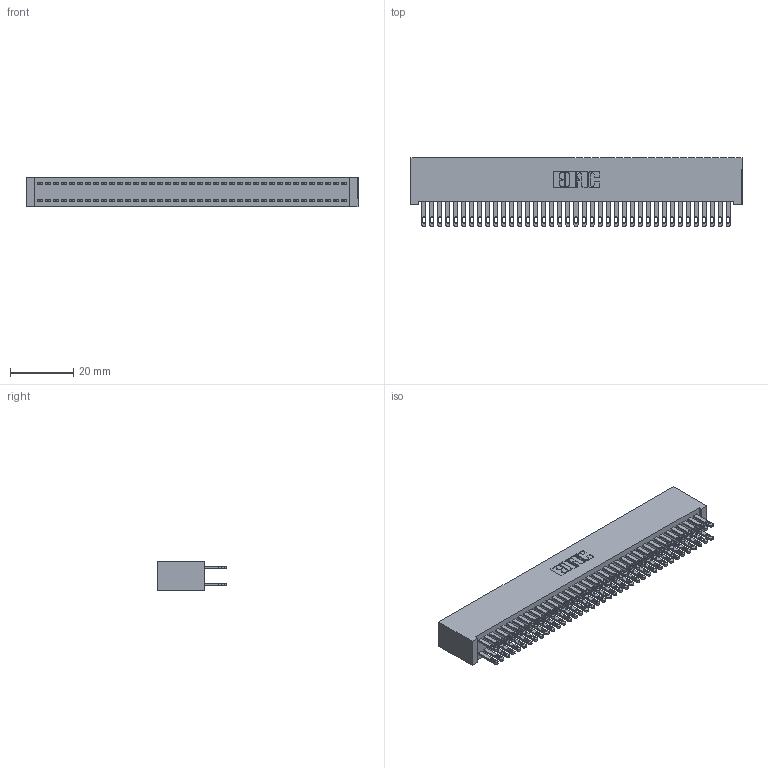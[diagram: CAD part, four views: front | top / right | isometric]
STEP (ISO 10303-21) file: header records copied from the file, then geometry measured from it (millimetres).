
FILE_DESCRIPTION (( 'STEP AP203' ), '1' );
FILE_NAME ('342-078-500-201.STEP', '2018-08-13T12:59:23', ( '' ), ( '' ), 'SwSTEP 2.0', 'SolidWorks 2016', '' );
FILE_SCHEMA (( 'CONFIG_CONTROL_DESIGN' ));
Length unit declared in the file: inch
Products named in the file (3): 342 Part_Lugless; 345-292-001_345-293-100; 342-078-500-201
Assembly tree (79 placements, depth 2):
  342-078-500-201
    342 Part_Lugless
    345-292-001_345-293-100  x78
Bounding box: 105.31 x 21.85 x 9.4 mm (x, y, z)
Volume: 10125.6 mm3; surface area: 17601.1 mm2
Topology: 79 solids, 79 shells, 3846 faces, 11741 edges, 7826 vertices
Faces by surface type: plane 2402, cylinder 1444
Entity records: 24999 total; most frequent: CARTESIAN_POINT 4142, ORIENTED_EDGE 4078, DIRECTION 3539, EDGE_CURVE 2039, VECTOR 1915, LINE 1915, VERTEX_POINT 1358, AXIS2_PLACEMENT_3D 812
